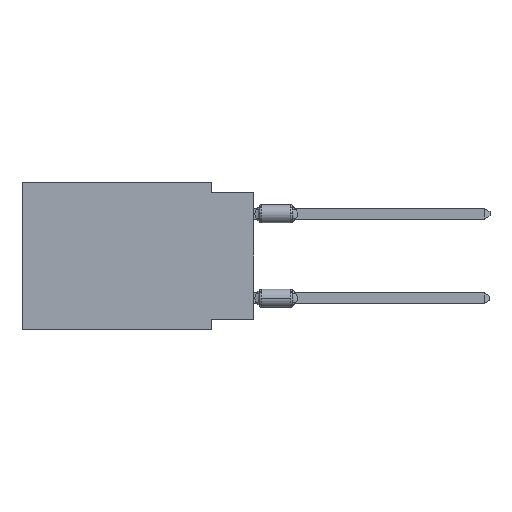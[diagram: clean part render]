
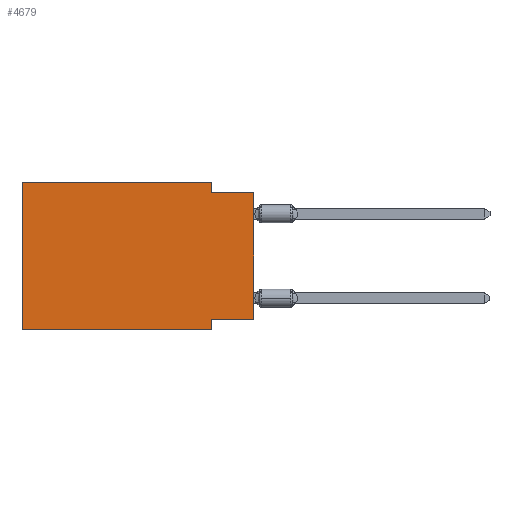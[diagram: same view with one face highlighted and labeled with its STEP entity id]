
A CAD part, left-side view. The second image highlights one B-rep face of the part: STEP entity #4679.
In plain terms, the highlighted planar face has unit normal (-1, 0, 0).
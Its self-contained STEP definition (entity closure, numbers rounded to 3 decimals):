
#242 = VERTEX_POINT ( 'NONE', #12587 ) ;
#260 = DIRECTION ( 'NONE',  ( 0., 0., -1. ) ) ;
#363 = EDGE_CURVE ( 'NONE', #2944, #4584, #11569, .T. ) ;
#389 = ORIENTED_EDGE ( 'NONE', *, *, #1386, .F. ) ;
#722 = DIRECTION ( 'NONE',  ( 0., 0., -1. ) ) ;
#773 = AXIS2_PLACEMENT_3D ( 'NONE', #4960, #14882, #722 ) ;
#806 = CARTESIAN_POINT ( 'NONE',  ( 0., 2.54, -8.89 ) ) ;
#1386 = EDGE_CURVE ( 'NONE', #3135, #4584, #2963, .T. ) ;
#1741 = CARTESIAN_POINT ( 'NONE',  ( 0., 2.54, -0.635 ) ) ;
#1987 = VECTOR ( 'NONE', #2589, 1000. ) ;
#2512 = LINE ( 'NONE', #6503, #8791 ) ;
#2589 = DIRECTION ( 'NONE',  ( 0., -1., 0. ) ) ;
#2624 = ORIENTED_EDGE ( 'NONE', *, *, #363, .T. ) ;
#2944 = VERTEX_POINT ( 'NONE', #5409 ) ;
#2947 = VERTEX_POINT ( 'NONE', #5751 ) ;
#2963 = LINE ( 'NONE', #8221, #9552 ) ;
#3135 = VERTEX_POINT ( 'NONE', #9972 ) ;
#3234 = EDGE_CURVE ( 'NONE', #242, #13552, #2512, .T. ) ;
#3819 = VECTOR ( 'NONE', #16540, 1000. ) ;
#3965 = DIRECTION ( 'NONE',  ( 0., 1., 0. ) ) ;
#4086 = VECTOR ( 'NONE', #12410, 1000. ) ;
#4369 = VERTEX_POINT ( 'NONE', #11825 ) ;
#4584 = VERTEX_POINT ( 'NONE', #806 ) ;
#4625 = CARTESIAN_POINT ( 'NONE',  ( 0., 13.97, 0. ) ) ;
#4679 = ADVANCED_FACE ( 'NONE', ( #6230 ), #8522, .F. ) ;
#4960 = CARTESIAN_POINT ( 'NONE',  ( 0., 13.97, 0. ) ) ;
#5185 = CARTESIAN_POINT ( 'NONE',  ( 0., 0., 0. ) ) ;
#5409 = CARTESIAN_POINT ( 'NONE',  ( 0., 13.97, -8.89 ) ) ;
#5549 = CARTESIAN_POINT ( 'NONE',  ( 0., 2.54, 0. ) ) ;
#5621 = VERTEX_POINT ( 'NONE', #1741 ) ;
#5751 = CARTESIAN_POINT ( 'NONE',  ( 0., 0., -8.255 ) ) ;
#6193 = LINE ( 'NONE', #11357, #3819 ) ;
#6230 = FACE_OUTER_BOUND ( 'NONE', #6755, .T. ) ;
#6417 = ORIENTED_EDGE ( 'NONE', *, *, #3234, .F. ) ;
#6503 = CARTESIAN_POINT ( 'NONE',  ( 0., 13.97, 0. ) ) ;
#6755 = EDGE_LOOP ( 'NONE', ( #15939, #9896, #8760, #6417, #10343, #2624, #389, #15010 ) ) ;
#6765 = EDGE_CURVE ( 'NONE', #5621, #4369, #6193, .T. ) ;
#6796 = EDGE_CURVE ( 'NONE', #2947, #4369, #11608, .T. ) ;
#8221 = CARTESIAN_POINT ( 'NONE',  ( 0., 2.54, -8.89 ) ) ;
#8522 = PLANE ( 'NONE',  #773 ) ;
#8760 = ORIENTED_EDGE ( 'NONE', *, *, #10121, .F. ) ;
#8791 = VECTOR ( 'NONE', #12673, 1000. ) ;
#9199 = CARTESIAN_POINT ( 'NONE',  ( 0., 13.97, -8.89 ) ) ;
#9240 = VECTOR ( 'NONE', #14516, 1000. ) ;
#9433 = CARTESIAN_POINT ( 'NONE',  ( 0., 2.54, 0. ) ) ;
#9552 = VECTOR ( 'NONE', #260, 1000. ) ;
#9796 = EDGE_CURVE ( 'NONE', #2944, #242, #12653, .T. ) ;
#9896 = ORIENTED_EDGE ( 'NONE', *, *, #6765, .F. ) ;
#9972 = CARTESIAN_POINT ( 'NONE',  ( 0., 2.54, -8.255 ) ) ;
#10121 = EDGE_CURVE ( 'NONE', #13552, #5621, #10951, .T. ) ;
#10343 = ORIENTED_EDGE ( 'NONE', *, *, #9796, .F. ) ;
#10951 = LINE ( 'NONE', #9433, #9240 ) ;
#11357 = CARTESIAN_POINT ( 'NONE',  ( 0., 0., -0.635 ) ) ;
#11423 = CARTESIAN_POINT ( 'NONE',  ( 0., 0., -8.255 ) ) ;
#11569 = LINE ( 'NONE', #9199, #1987 ) ;
#11608 = LINE ( 'NONE', #5185, #13556 ) ;
#11825 = CARTESIAN_POINT ( 'NONE',  ( 0., 0., -0.635 ) ) ;
#12410 = DIRECTION ( 'NONE',  ( 0., 0., 1. ) ) ;
#12587 = CARTESIAN_POINT ( 'NONE',  ( 0., 13.97, 0. ) ) ;
#12653 = LINE ( 'NONE', #4625, #4086 ) ;
#12673 = DIRECTION ( 'NONE',  ( 0., -1., 0. ) ) ;
#13552 = VERTEX_POINT ( 'NONE', #5549 ) ;
#13556 = VECTOR ( 'NONE', #15518, 1000. ) ;
#14055 = LINE ( 'NONE', #11423, #15124 ) ;
#14516 = DIRECTION ( 'NONE',  ( 0., 0., -1. ) ) ;
#14619 = EDGE_CURVE ( 'NONE', #2947, #3135, #14055, .T. ) ;
#14882 = DIRECTION ( 'NONE',  ( 1., 0., 0. ) ) ;
#15010 = ORIENTED_EDGE ( 'NONE', *, *, #14619, .F. ) ;
#15124 = VECTOR ( 'NONE', #3965, 1000. ) ;
#15518 = DIRECTION ( 'NONE',  ( 0., 0., 1. ) ) ;
#15939 = ORIENTED_EDGE ( 'NONE', *, *, #6796, .T. ) ;
#16540 = DIRECTION ( 'NONE',  ( 0., -1., 0. ) ) ;
